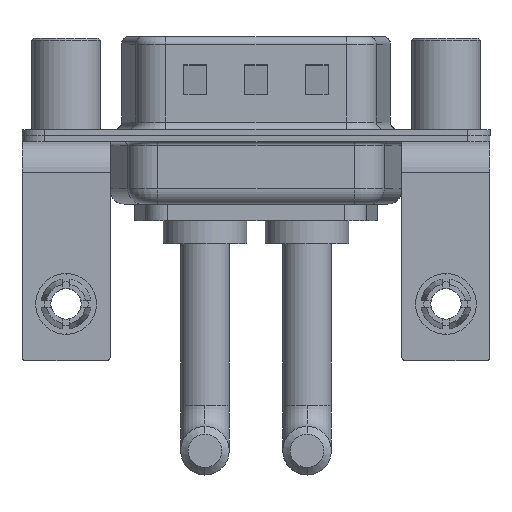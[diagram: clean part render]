
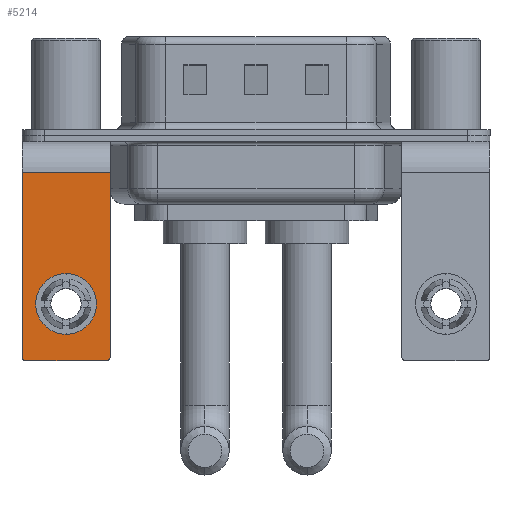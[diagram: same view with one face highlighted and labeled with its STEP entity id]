
A CAD part, front view. The second image highlights one B-rep face of the part: STEP entity #5214.
In plain terms, the highlighted planar face has unit normal (0, -1, 0).
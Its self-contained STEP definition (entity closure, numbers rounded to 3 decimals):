
#20 = VERTEX_POINT ( 'NONE', #13469 ) ;
#182 = CARTESIAN_POINT ( 'NONE',  ( 0., -6.25, -11.07 ) ) ;
#212 = DIRECTION ( 'NONE',  ( 0., 0., -1. ) ) ;
#306 = DIRECTION ( 'NONE',  ( -1., 0., 0. ) ) ;
#703 = VERTEX_POINT ( 'NONE', #18327 ) ;
#1098 = AXIS2_PLACEMENT_3D ( 'NONE', #9150, #7752, #5133 ) ;
#1137 = ORIENTED_EDGE ( 'NONE', *, *, #11379, .T. ) ;
#1150 = VERTEX_POINT ( 'NONE', #6964 ) ;
#1191 = VECTOR ( 'NONE', #212, 1000. ) ;
#1247 = EDGE_CURVE ( 'NONE', #8692, #1150, #14690, .T. ) ;
#1309 = DIRECTION ( 'NONE',  ( 0., 0., 1. ) ) ;
#1577 = DIRECTION ( 'NONE',  ( 0., 1., 0. ) ) ;
#1886 = CARTESIAN_POINT ( 'NONE',  ( 0., -6.25, -11.07 ) ) ;
#1975 = DIRECTION ( 'NONE',  ( 0., 0., 1. ) ) ;
#2134 = EDGE_CURVE ( 'NONE', #10479, #17256, #13148, .T. ) ;
#2279 = ORIENTED_EDGE ( 'NONE', *, *, #2769, .T. ) ;
#2676 = CIRCLE ( 'NONE', #8055, 2. ) ;
#2769 = EDGE_CURVE ( 'NONE', #8692, #5411, #17076, .T. ) ;
#3091 = DIRECTION ( 'NONE',  ( 0., 0., -1. ) ) ;
#3238 = AXIS2_PLACEMENT_3D ( 'NONE', #182, #1577, #1309 ) ;
#3919 = AXIS2_PLACEMENT_3D ( 'NONE', #16829, #9705, #15413 ) ;
#4356 = VERTEX_POINT ( 'NONE', #16076 ) ;
#4852 = AXIS2_PLACEMENT_3D ( 'NONE', #13884, #6892, #12480 ) ;
#5133 = DIRECTION ( 'NONE',  ( 0., 0., 1. ) ) ;
#5171 = ORIENTED_EDGE ( 'NONE', *, *, #1247, .F. ) ;
#5214 = ADVANCED_FACE ( 'NONE', ( #5474, #5654 ), #8191, .F. ) ;
#5411 = VERTEX_POINT ( 'NONE', #16216 ) ;
#5474 = FACE_BOUND ( 'NONE', #8421, .T. ) ;
#5654 = FACE_OUTER_BOUND ( 'NONE', #14010, .T. ) ;
#5810 = DIRECTION ( 'NONE',  ( 0., 1., 0. ) ) ;
#6892 = DIRECTION ( 'NONE',  ( 0., 1., 0. ) ) ;
#6919 = VECTOR ( 'NONE', #16028, 1000. ) ;
#6964 = CARTESIAN_POINT ( 'NONE',  ( 2.9, -6.25, -14.55 ) ) ;
#7752 = DIRECTION ( 'NONE',  ( 0., -1., 0. ) ) ;
#8055 = AXIS2_PLACEMENT_3D ( 'NONE', #1886, #5810, #1975 ) ;
#8191 = PLANE ( 'NONE',  #4852 ) ;
#8228 = EDGE_CURVE ( 'NONE', #5411, #10479, #11509, .T. ) ;
#8315 = CIRCLE ( 'NONE', #3238, 2. ) ;
#8421 = EDGE_LOOP ( 'NONE', ( #17172, #1137 ) ) ;
#8692 = VERTEX_POINT ( 'NONE', #9195 ) ;
#8867 = VECTOR ( 'NONE', #306, 1000. ) ;
#8993 = CARTESIAN_POINT ( 'NONE',  ( 2.9, -6.25, -14.8 ) ) ;
#9114 = VECTOR ( 'NONE', #3091, 1000. ) ;
#9139 = EDGE_CURVE ( 'NONE', #703, #1150, #9161, .T. ) ;
#9150 = CARTESIAN_POINT ( 'NONE',  ( 2.65, -6.25, -14.55 ) ) ;
#9161 = CIRCLE ( 'NONE', #1098, 0.25 ) ;
#9195 = CARTESIAN_POINT ( 'NONE',  ( 2.9, -6.25, -2.4 ) ) ;
#9705 = DIRECTION ( 'NONE',  ( 0., -1., 0. ) ) ;
#9907 = ORIENTED_EDGE ( 'NONE', *, *, #9139, .T. ) ;
#10194 = CARTESIAN_POINT ( 'NONE',  ( -2.9, -6.25, -2.4 ) ) ;
#10321 = CARTESIAN_POINT ( 'NONE',  ( 2.9, -6.25, -2.4 ) ) ;
#10479 = VERTEX_POINT ( 'NONE', #12640 ) ;
#10511 = EDGE_CURVE ( 'NONE', #703, #17256, #14595, .T. ) ;
#10692 = ORIENTED_EDGE ( 'NONE', *, *, #2134, .T. ) ;
#11379 = EDGE_CURVE ( 'NONE', #20, #4356, #8315, .T. ) ;
#11509 = LINE ( 'NONE', #10194, #9114 ) ;
#11892 = CARTESIAN_POINT ( 'NONE',  ( 2.9, -6.25, -2.4 ) ) ;
#12480 = DIRECTION ( 'NONE',  ( 0., 0., 1. ) ) ;
#12640 = CARTESIAN_POINT ( 'NONE',  ( -2.9, -6.25, -14.55 ) ) ;
#13148 = CIRCLE ( 'NONE', #3919, 0.25 ) ;
#13469 = CARTESIAN_POINT ( 'NONE',  ( 0., -6.25, -9.07 ) ) ;
#13884 = CARTESIAN_POINT ( 'NONE',  ( 2.9, -6.25, -2.4 ) ) ;
#14010 = EDGE_LOOP ( 'NONE', ( #16311, #10692, #15007, #9907, #5171, #2279 ) ) ;
#14595 = LINE ( 'NONE', #8993, #8867 ) ;
#14690 = LINE ( 'NONE', #11892, #1191 ) ;
#15007 = ORIENTED_EDGE ( 'NONE', *, *, #10511, .F. ) ;
#15413 = DIRECTION ( 'NONE',  ( 0., 0., 1. ) ) ;
#16028 = DIRECTION ( 'NONE',  ( -1., 0., 0. ) ) ;
#16076 = CARTESIAN_POINT ( 'NONE',  ( 0., -6.25, -13.07 ) ) ;
#16087 = CARTESIAN_POINT ( 'NONE',  ( -2.65, -6.25, -14.8 ) ) ;
#16216 = CARTESIAN_POINT ( 'NONE',  ( -2.9, -6.25, -2.4 ) ) ;
#16311 = ORIENTED_EDGE ( 'NONE', *, *, #8228, .T. ) ;
#16829 = CARTESIAN_POINT ( 'NONE',  ( -2.65, -6.25, -14.55 ) ) ;
#17076 = LINE ( 'NONE', #10321, #6919 ) ;
#17172 = ORIENTED_EDGE ( 'NONE', *, *, #18418, .T. ) ;
#17256 = VERTEX_POINT ( 'NONE', #16087 ) ;
#18327 = CARTESIAN_POINT ( 'NONE',  ( 2.65, -6.25, -14.8 ) ) ;
#18418 = EDGE_CURVE ( 'NONE', #4356, #20, #2676, .T. ) ;
